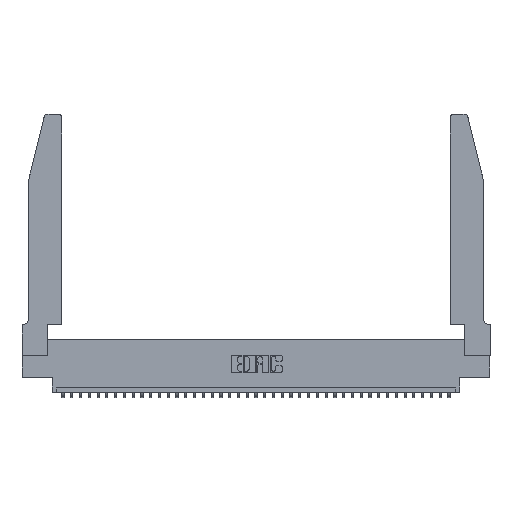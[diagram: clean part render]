
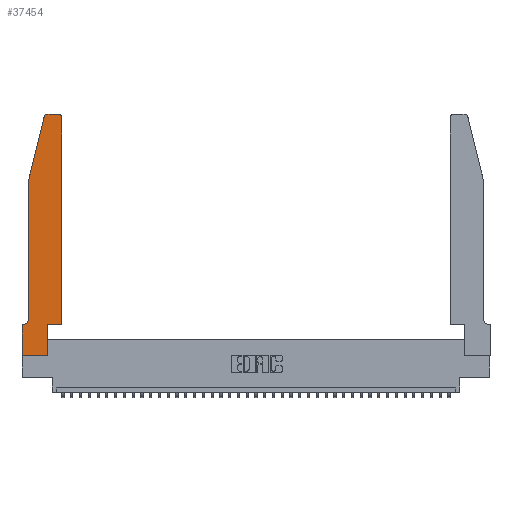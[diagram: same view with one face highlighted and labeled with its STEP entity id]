
A CAD part, top view. The second image highlights one B-rep face of the part: STEP entity #37454.
In plain terms, the highlighted planar face has unit normal (0, 0, 1).
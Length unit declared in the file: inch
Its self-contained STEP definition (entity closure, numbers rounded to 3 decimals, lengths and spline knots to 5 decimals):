
#978 = ORIENTED_EDGE ( 'NONE', *, *, #21080, .T. ) ;
#1233 = ORIENTED_EDGE ( 'NONE', *, *, #10462, .T. ) ;
#1345 = VERTEX_POINT ( 'NONE', #6495 ) ;
#2090 = VECTOR ( 'NONE', #3713, 39.37008 ) ;
#2599 = DIRECTION ( 'NONE',  ( 1., 0., 0. ) ) ;
#2708 = ORIENTED_EDGE ( 'NONE', *, *, #16557, .T. ) ;
#2866 = ORIENTED_EDGE ( 'NONE', *, *, #26163, .T. ) ;
#2887 = CARTESIAN_POINT ( 'NONE',  ( 0., 0.35, 0.37 ) ) ;
#3034 = CARTESIAN_POINT ( 'NONE',  ( 0.4505, 2.72, 0.37 ) ) ;
#3713 = DIRECTION ( 'NONE',  ( -1., 0., 0. ) ) ;
#4039 = ORIENTED_EDGE ( 'NONE', *, *, #25929, .T. ) ;
#4829 = DIRECTION ( 'NONE',  ( 0., 0., 1. ) ) ;
#5178 = CIRCLE ( 'NONE', #22228, 0.07 ) ;
#5363 = VECTOR ( 'NONE', #13244, 39.37008 ) ;
#5762 = ORIENTED_EDGE ( 'NONE', *, *, #14466, .T. ) ;
#5856 = VECTOR ( 'NONE', #15482, 39.37008 ) ;
#6055 = CARTESIAN_POINT ( 'NONE',  ( 0.0055, 0.35, 0.37 ) ) ;
#6407 = CARTESIAN_POINT ( 'NONE',  ( 0.0755, 2., 0.37 ) ) ;
#6495 = CARTESIAN_POINT ( 'NONE',  ( 0.4205, 2.75, 0.37 ) ) ;
#7179 = CIRCLE ( 'NONE', #7326, 0.03 ) ;
#7326 = AXIS2_PLACEMENT_3D ( 'NONE', #37253, #14029, #34543 ) ;
#7837 = DIRECTION ( 'NONE',  ( -1., 0., 0. ) ) ;
#7964 = CARTESIAN_POINT ( 'NONE',  ( 0.0755, 2., 0.37 ) ) ;
#9034 = CARTESIAN_POINT ( 'NONE',  ( 0.0755, 2., 0.37 ) ) ;
#9310 = VECTOR ( 'NONE', #37198, 39.37008 ) ;
#9605 = CARTESIAN_POINT ( 'NONE',  ( 0.4505, 0.35, 0.37 ) ) ;
#10362 = ORIENTED_EDGE ( 'NONE', *, *, #12978, .T. ) ;
#10462 = EDGE_CURVE ( 'NONE', #1345, #26403, #37365, .T. ) ;
#10562 = AXIS2_PLACEMENT_3D ( 'NONE', #12967, #18812, #21760 ) ;
#11061 = AXIS2_PLACEMENT_3D ( 'NONE', #33893, #4829, #31490 ) ;
#11205 = EDGE_CURVE ( 'NONE', #13946, #16946, #29016, .T. ) ;
#12461 = ORIENTED_EDGE ( 'NONE', *, *, #29993, .T. ) ;
#12468 = VERTEX_POINT ( 'NONE', #9605 ) ;
#12967 = CARTESIAN_POINT ( 'NONE',  ( 0.284, 2.72, 0.37 ) ) ;
#12978 = EDGE_CURVE ( 'NONE', #27762, #24547, #5178, .T. ) ;
#13244 = DIRECTION ( 'NONE',  ( 0., -1., 0. ) ) ;
#13349 = LINE ( 'NONE', #25040, #5363 ) ;
#13946 = VERTEX_POINT ( 'NONE', #17450 ) ;
#14029 = DIRECTION ( 'NONE',  ( 0., 0., 1. ) ) ;
#14248 = CARTESIAN_POINT ( 'NONE',  ( 0., 0., 0.37 ) ) ;
#14456 = ORIENTED_EDGE ( 'NONE', *, *, #11205, .T. ) ;
#14466 = EDGE_CURVE ( 'NONE', #20693, #21145, #19623, .T. ) ;
#14614 = ORIENTED_EDGE ( 'NONE', *, *, #34422, .T. ) ;
#15482 = DIRECTION ( 'NONE',  ( 0., -1., 0. ) ) ;
#16557 = EDGE_CURVE ( 'NONE', #16946, #27762, #17127, .T. ) ;
#16855 = FACE_OUTER_BOUND ( 'NONE', #35095, .T. ) ;
#16946 = VERTEX_POINT ( 'NONE', #6407 ) ;
#17127 = LINE ( 'NONE', #7964, #5856 ) ;
#17230 = CARTESIAN_POINT ( 'NONE',  ( 0.0755, 0.35, 0.37 ) ) ;
#17450 = CARTESIAN_POINT ( 'NONE',  ( 0.25487, 2.72718, 0.37 ) ) ;
#18812 = DIRECTION ( 'NONE',  ( 0., 0., 1. ) ) ;
#18825 = VECTOR ( 'NONE', #19032, 39.37008 ) ;
#18931 = CARTESIAN_POINT ( 'NONE',  ( 0.284, 2.75, 0.37 ) ) ;
#19032 = DIRECTION ( 'NONE',  ( 0., 1., 0. ) ) ;
#19623 = LINE ( 'NONE', #14248, #28826 ) ;
#20183 = DIRECTION ( 'NONE',  ( -1., 0., 0. ) ) ;
#20580 = VECTOR ( 'NONE', #20183, 39.37008 ) ;
#20693 = VERTEX_POINT ( 'NONE', #33192 ) ;
#21080 = EDGE_CURVE ( 'NONE', #26403, #13946, #30843, .T. ) ;
#21135 = VECTOR ( 'NONE', #29527, 39.37008 ) ;
#21145 = VERTEX_POINT ( 'NONE', #30809 ) ;
#21454 = LINE ( 'NONE', #17230, #20580 ) ;
#21760 = DIRECTION ( 'NONE',  ( 1., 0., 0. ) ) ;
#22094 = CARTESIAN_POINT ( 'NONE',  ( 0.4505, 0.35, 0.37 ) ) ;
#22228 = AXIS2_PLACEMENT_3D ( 'NONE', #25042, #28899, #7837 ) ;
#22717 = PLANE ( 'NONE',  #11061 ) ;
#24547 = VERTEX_POINT ( 'NONE', #6055 ) ;
#24662 = CARTESIAN_POINT ( 'NONE',  ( 0.2605, 2.75, 0.37 ) ) ;
#25040 = CARTESIAN_POINT ( 'NONE',  ( 0., 0., 0.37 ) ) ;
#25042 = CARTESIAN_POINT ( 'NONE',  ( 0.0055, 0.42, 0.37 ) ) ;
#25929 = EDGE_CURVE ( 'NONE', #24547, #35167, #21454, .T. ) ;
#26163 = EDGE_CURVE ( 'NONE', #12468, #32800, #32586, .T. ) ;
#26403 = VERTEX_POINT ( 'NONE', #18931 ) ;
#27374 = EDGE_CURVE ( 'NONE', #31637, #12468, #37601, .T. ) ;
#27762 = VERTEX_POINT ( 'NONE', #33038 ) ;
#28539 = LINE ( 'NONE', #31294, #18825 ) ;
#28826 = VECTOR ( 'NONE', #2599, 39.37008 ) ;
#28899 = DIRECTION ( 'NONE',  ( 0., 0., -1. ) ) ;
#29016 = LINE ( 'NONE', #9034, #21135 ) ;
#29527 = DIRECTION ( 'NONE',  ( -0.239, -0.971, 0. ) ) ;
#29993 = EDGE_CURVE ( 'NONE', #32800, #1345, #7179, .T. ) ;
#30547 = EDGE_CURVE ( 'NONE', #21145, #31637, #28539, .T. ) ;
#30809 = CARTESIAN_POINT ( 'NONE',  ( 0.2865, 0., 0.37 ) ) ;
#30843 = CIRCLE ( 'NONE', #10562, 0.03 ) ;
#31265 = CARTESIAN_POINT ( 'NONE',  ( 0.4505, 0.35, 0.37 ) ) ;
#31294 = CARTESIAN_POINT ( 'NONE',  ( 0.2865, 0.35, 0.37 ) ) ;
#31490 = DIRECTION ( 'NONE',  ( 1., 0., 0. ) ) ;
#31637 = VERTEX_POINT ( 'NONE', #33368 ) ;
#32586 = LINE ( 'NONE', #31265, #36683 ) ;
#32800 = VERTEX_POINT ( 'NONE', #3034 ) ;
#33038 = CARTESIAN_POINT ( 'NONE',  ( 0.0755, 0.42, 0.37 ) ) ;
#33192 = CARTESIAN_POINT ( 'NONE',  ( 0., 0., 0.37 ) ) ;
#33368 = CARTESIAN_POINT ( 'NONE',  ( 0.2865, 0.35, 0.37 ) ) ;
#33702 = ORIENTED_EDGE ( 'NONE', *, *, #27374, .T. ) ;
#33893 = CARTESIAN_POINT ( 'NONE',  ( 0., 0.35, 0.37 ) ) ;
#34071 = ORIENTED_EDGE ( 'NONE', *, *, #30547, .T. ) ;
#34422 = EDGE_CURVE ( 'NONE', #35167, #20693, #13349, .T. ) ;
#34543 = DIRECTION ( 'NONE',  ( 1., 0., 0. ) ) ;
#35095 = EDGE_LOOP ( 'NONE', ( #1233, #978, #14456, #2708, #10362, #4039, #14614, #5762, #34071, #33702, #2866, #12461 ) ) ;
#35167 = VERTEX_POINT ( 'NONE', #2887 ) ;
#36683 = VECTOR ( 'NONE', #37041, 39.37008 ) ;
#37041 = DIRECTION ( 'NONE',  ( 0., 1., 0. ) ) ;
#37198 = DIRECTION ( 'NONE',  ( 1., 0., 0. ) ) ;
#37253 = CARTESIAN_POINT ( 'NONE',  ( 0.4205, 2.72, 0.37 ) ) ;
#37365 = LINE ( 'NONE', #24662, #2090 ) ;
#37454 = ADVANCED_FACE ( 'NONE', ( #16855 ), #22717, .T. ) ;
#37601 = LINE ( 'NONE', #22094, #9310 ) ;
